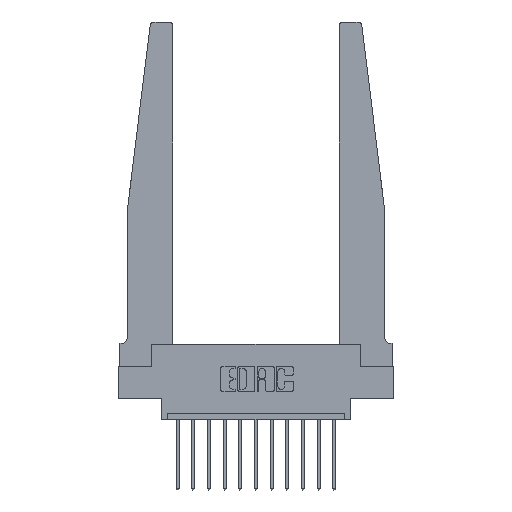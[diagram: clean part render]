
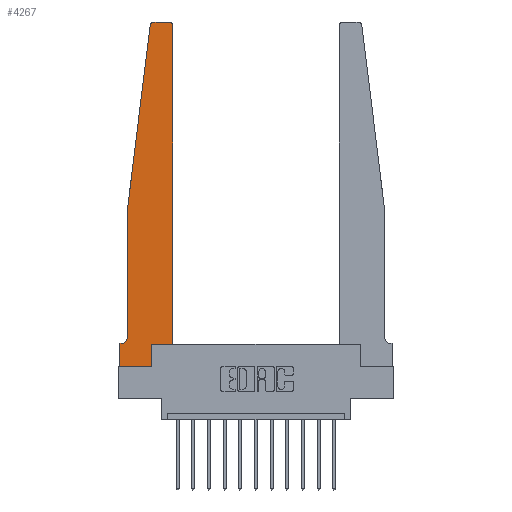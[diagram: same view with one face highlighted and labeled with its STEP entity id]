
A CAD part, top view. The second image highlights one B-rep face of the part: STEP entity #4267.
In plain terms, the highlighted planar face has unit normal (0, 0, 1).
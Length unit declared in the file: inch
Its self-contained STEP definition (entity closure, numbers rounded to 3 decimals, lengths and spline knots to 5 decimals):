
#52 = ORIENTED_EDGE ( 'NONE', *, *, #1979, .T. ) ;
#195 = DIRECTION ( 'NONE',  ( 0., 0., -1. ) ) ;
#440 = VECTOR ( 'NONE', #14381, 39.37008 ) ;
#485 = CARTESIAN_POINT ( 'NONE',  ( 0.27653, 2.72, 0.37 ) ) ;
#520 = DIRECTION ( 'NONE',  ( 1., 0., 0. ) ) ;
#575 = AXIS2_PLACEMENT_3D ( 'NONE', #7117, #12175, #16042 ) ;
#748 = EDGE_CURVE ( 'NONE', #1117, #6314, #7178, .T. ) ;
#1117 = VERTEX_POINT ( 'NONE', #9268 ) ;
#1392 = CARTESIAN_POINT ( 'NONE',  ( 0.065, 1.25, 0.37 ) ) ;
#1481 = DIRECTION ( 'NONE',  ( -0.122, -0.992, 0. ) ) ;
#1745 = CARTESIAN_POINT ( 'NONE',  ( 0.25, 2.75, 0.37 ) ) ;
#1979 = EDGE_CURVE ( 'NONE', #14727, #10176, #2033, .T. ) ;
#2026 = VERTEX_POINT ( 'NONE', #16048 ) ;
#2033 = LINE ( 'NONE', #3096, #9667 ) ;
#2373 = DIRECTION ( 'NONE',  ( -1., 0., 0. ) ) ;
#2527 = DIRECTION ( 'NONE',  ( 0., -1., 0. ) ) ;
#2830 = EDGE_CURVE ( 'NONE', #10322, #5117, #10735, .T. ) ;
#2923 = ORIENTED_EDGE ( 'NONE', *, *, #14071, .T. ) ;
#2991 = CARTESIAN_POINT ( 'NONE',  ( 0.425, 0.18, 0.37 ) ) ;
#3096 = CARTESIAN_POINT ( 'NONE',  ( 0.425, 0.18, 0.37 ) ) ;
#3150 = LINE ( 'NONE', #2991, #7716 ) ;
#3285 = CARTESIAN_POINT ( 'NONE',  ( 0.065, 0.1875, 0.37 ) ) ;
#3307 = CARTESIAN_POINT ( 'NONE',  ( 0.065, 1.25, 0.37 ) ) ;
#3361 = ORIENTED_EDGE ( 'NONE', *, *, #5939, .T. ) ;
#3510 = VECTOR ( 'NONE', #2527, 39.37008 ) ;
#3679 = DIRECTION ( 'NONE',  ( 1., 0., 0. ) ) ;
#3705 = VERTEX_POINT ( 'NONE', #8440 ) ;
#3942 = EDGE_CURVE ( 'NONE', #2026, #7266, #4209, .T. ) ;
#4020 = EDGE_CURVE ( 'NONE', #5117, #10609, #9472, .T. ) ;
#4110 = CARTESIAN_POINT ( 'NONE',  ( 0., 0.1875, 0.37 ) ) ;
#4209 = LINE ( 'NONE', #3307, #10000 ) ;
#4267 = ADVANCED_FACE ( 'NONE', ( #11641 ), #10400, .T. ) ;
#4301 = DIRECTION ( 'NONE',  ( 0., 1., 0. ) ) ;
#4424 = DIRECTION ( 'NONE',  ( -1., 0., 0. ) ) ;
#4467 = AXIS2_PLACEMENT_3D ( 'NONE', #4110, #9146, #7588 ) ;
#4791 = ORIENTED_EDGE ( 'NONE', *, *, #7075, .T. ) ;
#4916 = CARTESIAN_POINT ( 'NONE',  ( 0.395, 2.75, 0.37 ) ) ;
#5117 = VERTEX_POINT ( 'NONE', #7747 ) ;
#5542 = DIRECTION ( 'NONE',  ( 1., 0., 0. ) ) ;
#5721 = CARTESIAN_POINT ( 'NONE',  ( 0.2605, 0.18, 0.37 ) ) ;
#5939 = EDGE_CURVE ( 'NONE', #10516, #14727, #6203, .T. ) ;
#5999 = LINE ( 'NONE', #3285, #12367 ) ;
#6203 = LINE ( 'NONE', #15374, #13501 ) ;
#6261 = CARTESIAN_POINT ( 'NONE',  ( 0., 0., 0.37 ) ) ;
#6314 = VERTEX_POINT ( 'NONE', #6261 ) ;
#6337 = ORIENTED_EDGE ( 'NONE', *, *, #8937, .T. ) ;
#6403 = LINE ( 'NONE', #1392, #14326 ) ;
#6414 = VECTOR ( 'NONE', #3679, 39.37008 ) ;
#7075 = EDGE_CURVE ( 'NONE', #14186, #10322, #8743, .T. ) ;
#7117 = CARTESIAN_POINT ( 'NONE',  ( 0.395, 2.72, 0.37 ) ) ;
#7178 = LINE ( 'NONE', #13852, #3510 ) ;
#7264 = EDGE_CURVE ( 'NONE', #10176, #14186, #3150, .T. ) ;
#7266 = VERTEX_POINT ( 'NONE', #14541 ) ;
#7302 = CIRCLE ( 'NONE', #12574, 0.05 ) ;
#7534 = DIRECTION ( 'NONE',  ( 0., 1., 0. ) ) ;
#7588 = DIRECTION ( 'NONE',  ( 1., 0., 0. ) ) ;
#7716 = VECTOR ( 'NONE', #4301, 39.37008 ) ;
#7747 = CARTESIAN_POINT ( 'NONE',  ( 0.27653, 2.75, 0.37 ) ) ;
#8001 = EDGE_CURVE ( 'NONE', #7266, #3705, #7302, .T. ) ;
#8440 = CARTESIAN_POINT ( 'NONE',  ( 0.015, 0.1875, 0.37 ) ) ;
#8743 = CIRCLE ( 'NONE', #575, 0.03 ) ;
#8937 = EDGE_CURVE ( 'NONE', #3705, #1117, #5999, .T. ) ;
#9146 = DIRECTION ( 'NONE',  ( 0., 0., 1. ) ) ;
#9236 = ORIENTED_EDGE ( 'NONE', *, *, #9827, .T. ) ;
#9268 = CARTESIAN_POINT ( 'NONE',  ( 0., 0.1875, 0.37 ) ) ;
#9341 = DIRECTION ( 'NONE',  ( 0., 0., 1. ) ) ;
#9472 = CIRCLE ( 'NONE', #11586, 0.03 ) ;
#9667 = VECTOR ( 'NONE', #520, 39.37008 ) ;
#9827 = EDGE_CURVE ( 'NONE', #10609, #2026, #6403, .T. ) ;
#10000 = VECTOR ( 'NONE', #14295, 39.37008 ) ;
#10007 = ORIENTED_EDGE ( 'NONE', *, *, #8001, .T. ) ;
#10176 = VERTEX_POINT ( 'NONE', #12285 ) ;
#10322 = VERTEX_POINT ( 'NONE', #4916 ) ;
#10378 = ORIENTED_EDGE ( 'NONE', *, *, #748, .T. ) ;
#10400 = PLANE ( 'NONE',  #4467 ) ;
#10516 = VERTEX_POINT ( 'NONE', #15655 ) ;
#10609 = VERTEX_POINT ( 'NONE', #15972 ) ;
#10687 = ORIENTED_EDGE ( 'NONE', *, *, #4020, .T. ) ;
#10735 = LINE ( 'NONE', #1745, #440 ) ;
#11555 = CARTESIAN_POINT ( 'NONE',  ( 0.015, 0.2375, 0.37 ) ) ;
#11586 = AXIS2_PLACEMENT_3D ( 'NONE', #485, #9341, #5542 ) ;
#11641 = FACE_OUTER_BOUND ( 'NONE', #12606, .T. ) ;
#12175 = DIRECTION ( 'NONE',  ( 0., 0., 1. ) ) ;
#12285 = CARTESIAN_POINT ( 'NONE',  ( 0.425, 0.18, 0.37 ) ) ;
#12367 = VECTOR ( 'NONE', #4424, 39.37008 ) ;
#12574 = AXIS2_PLACEMENT_3D ( 'NONE', #11555, #195, #2373 ) ;
#12606 = EDGE_LOOP ( 'NONE', ( #15266, #10687, #9236, #12714, #10007, #6337, #10378, #2923, #3361, #52, #14938, #4791 ) ) ;
#12681 = CARTESIAN_POINT ( 'NONE',  ( 0., 0., 0.37 ) ) ;
#12714 = ORIENTED_EDGE ( 'NONE', *, *, #3942, .T. ) ;
#13501 = VECTOR ( 'NONE', #7534, 39.37008 ) ;
#13768 = LINE ( 'NONE', #12681, #6414 ) ;
#13852 = CARTESIAN_POINT ( 'NONE',  ( 0., 0., 0.37 ) ) ;
#14071 = EDGE_CURVE ( 'NONE', #6314, #10516, #13768, .T. ) ;
#14186 = VERTEX_POINT ( 'NONE', #15414 ) ;
#14295 = DIRECTION ( 'NONE',  ( 0., -1., 0. ) ) ;
#14326 = VECTOR ( 'NONE', #1481, 39.37008 ) ;
#14381 = DIRECTION ( 'NONE',  ( -1., 0., 0. ) ) ;
#14541 = CARTESIAN_POINT ( 'NONE',  ( 0.065, 0.2375, 0.37 ) ) ;
#14727 = VERTEX_POINT ( 'NONE', #5721 ) ;
#14938 = ORIENTED_EDGE ( 'NONE', *, *, #7264, .T. ) ;
#15266 = ORIENTED_EDGE ( 'NONE', *, *, #2830, .T. ) ;
#15374 = CARTESIAN_POINT ( 'NONE',  ( 0.2605, 0.18, 0.37 ) ) ;
#15414 = CARTESIAN_POINT ( 'NONE',  ( 0.425, 2.72, 0.37 ) ) ;
#15655 = CARTESIAN_POINT ( 'NONE',  ( 0.2605, 0., 0.37 ) ) ;
#15972 = CARTESIAN_POINT ( 'NONE',  ( 0.24675, 2.72367, 0.37 ) ) ;
#16042 = DIRECTION ( 'NONE',  ( 1., 0., 0. ) ) ;
#16048 = CARTESIAN_POINT ( 'NONE',  ( 0.065, 1.25, 0.37 ) ) ;
